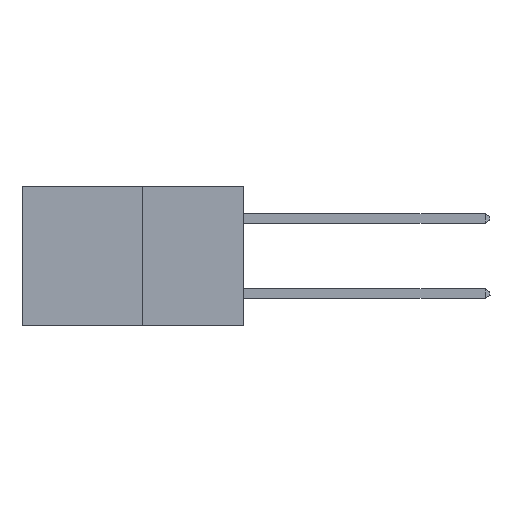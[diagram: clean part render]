
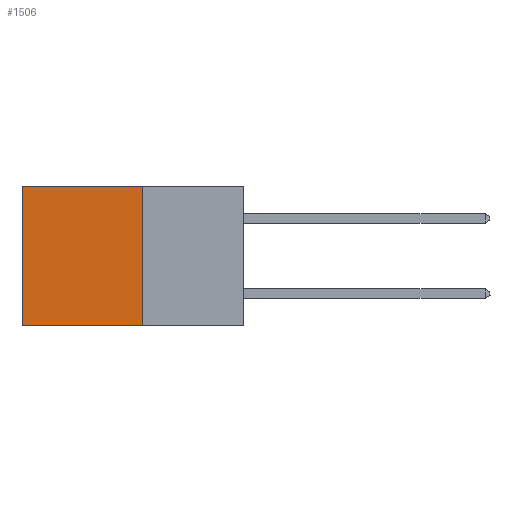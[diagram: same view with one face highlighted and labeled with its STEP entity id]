
A CAD part, left-side view. The second image highlights one B-rep face of the part: STEP entity #1506.
In plain terms, the highlighted planar face has unit normal (-1, 0, 0).
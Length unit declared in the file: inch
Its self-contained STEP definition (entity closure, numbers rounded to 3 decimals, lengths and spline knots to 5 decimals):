
#1444 = VERTEX_POINT ( 'NONE', #3637 ) ;
#1463 = PLANE ( 'NONE',  #7900 ) ;
#1506 = ADVANCED_FACE ( 'NONE', ( #14030 ), #1463, .F. ) ;
#2915 = VECTOR ( 'NONE', #22342, 39.37008 ) ;
#3476 = DIRECTION ( 'NONE',  ( 1., 0., 0. ) ) ;
#3637 = CARTESIAN_POINT ( 'NONE',  ( 0.277, 0.27, 0. ) ) ;
#4032 = ORIENTED_EDGE ( 'NONE', *, *, #6833, .T. ) ;
#5027 = VERTEX_POINT ( 'NONE', #16181 ) ;
#5870 = VECTOR ( 'NONE', #12795, 39.37008 ) ;
#6434 = LINE ( 'NONE', #21797, #5870 ) ;
#6688 = LINE ( 'NONE', #8747, #21646 ) ;
#6833 = EDGE_CURVE ( 'NONE', #1444, #22839, #6688, .T. ) ;
#7708 = LINE ( 'NONE', #15059, #2915 ) ;
#7900 = AXIS2_PLACEMENT_3D ( 'NONE', #10020, #3476, #22711 ) ;
#8747 = CARTESIAN_POINT ( 'NONE',  ( 0.277, 0.27, 0. ) ) ;
#9148 = DIRECTION ( 'NONE',  ( 0., 1., 0. ) ) ;
#10020 = CARTESIAN_POINT ( 'NONE',  ( 0.277, 0.27, -0.37 ) ) ;
#10132 = VERTEX_POINT ( 'NONE', #14508 ) ;
#10412 = ORIENTED_EDGE ( 'NONE', *, *, #10806, .F. ) ;
#10806 = EDGE_CURVE ( 'NONE', #10132, #5027, #15510, .T. ) ;
#12382 = ORIENTED_EDGE ( 'NONE', *, *, #16679, .T. ) ;
#12795 = DIRECTION ( 'NONE',  ( 0., 0., -1. ) ) ;
#13340 = EDGE_LOOP ( 'NONE', ( #12382, #10412, #16042, #4032 ) ) ;
#14030 = FACE_OUTER_BOUND ( 'NONE', #13340, .T. ) ;
#14392 = VECTOR ( 'NONE', #21759, 39.37008 ) ;
#14508 = CARTESIAN_POINT ( 'NONE',  ( 0.277, 0.27, -0.37 ) ) ;
#15059 = CARTESIAN_POINT ( 'NONE',  ( 0.277, 0.27, -0.37 ) ) ;
#15510 = LINE ( 'NONE', #16293, #14392 ) ;
#16042 = ORIENTED_EDGE ( 'NONE', *, *, #19328, .F. ) ;
#16181 = CARTESIAN_POINT ( 'NONE',  ( 0.277, 0.59, -0.37 ) ) ;
#16293 = CARTESIAN_POINT ( 'NONE',  ( 0.277, 0.27, -0.37 ) ) ;
#16679 = EDGE_CURVE ( 'NONE', #22839, #5027, #6434, .T. ) ;
#18529 = CARTESIAN_POINT ( 'NONE',  ( 0.277, 0.59, 0. ) ) ;
#19328 = EDGE_CURVE ( 'NONE', #1444, #10132, #7708, .T. ) ;
#21646 = VECTOR ( 'NONE', #9148, 39.37008 ) ;
#21759 = DIRECTION ( 'NONE',  ( 0., 1., 0. ) ) ;
#21797 = CARTESIAN_POINT ( 'NONE',  ( 0.277, 0.59, -0.37 ) ) ;
#22342 = DIRECTION ( 'NONE',  ( 0., 0., -1. ) ) ;
#22711 = DIRECTION ( 'NONE',  ( 0., 0., -1. ) ) ;
#22839 = VERTEX_POINT ( 'NONE', #18529 ) ;
